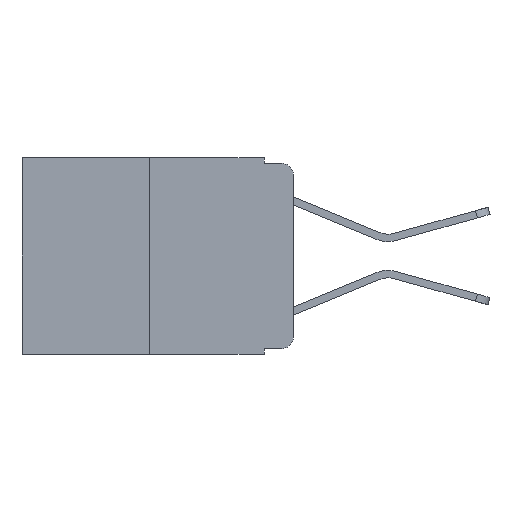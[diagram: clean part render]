
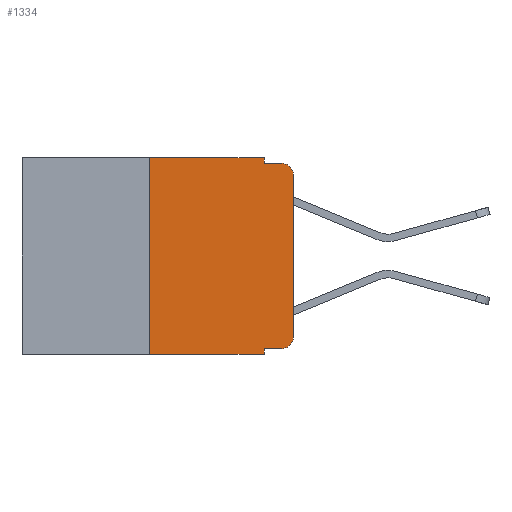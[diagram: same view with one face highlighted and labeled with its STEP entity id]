
A CAD part, left-side view. The second image highlights one B-rep face of the part: STEP entity #1334.
In plain terms, the highlighted planar face has unit normal (-1, 0, 0).
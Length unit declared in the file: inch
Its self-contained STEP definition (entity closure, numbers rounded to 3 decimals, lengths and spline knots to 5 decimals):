
#19 = VERTEX_POINT ( 'NONE', #2599 ) ;
#190 = EDGE_CURVE ( 'NONE', #11902, #3513, #4245, .T. ) ;
#820 = DIRECTION ( 'NONE',  ( 0., 0., 1. ) ) ;
#927 = LINE ( 'NONE', #3336, #10646 ) ;
#1154 = AXIS2_PLACEMENT_3D ( 'NONE', #10845, #9882, #5046 ) ;
#1334 = ADVANCED_FACE ( 'NONE', ( #6872 ), #12000, .F. ) ;
#1386 = ORIENTED_EDGE ( 'NONE', *, *, #3109, .F. ) ;
#1428 = CARTESIAN_POINT ( 'NONE',  ( 0., 0.02, -0.01 ) ) ;
#1674 = VECTOR ( 'NONE', #9749, 39.37008 ) ;
#1678 = CARTESIAN_POINT ( 'NONE',  ( 0., 0.051, -0.343 ) ) ;
#1734 = LINE ( 'NONE', #8211, #8474 ) ;
#1863 = CARTESIAN_POINT ( 'NONE',  ( 0., 0., 0. ) ) ;
#2050 = ORIENTED_EDGE ( 'NONE', *, *, #190, .T. ) ;
#2599 = CARTESIAN_POINT ( 'NONE',  ( 0., 0.051, -0.01 ) ) ;
#2748 = ORIENTED_EDGE ( 'NONE', *, *, #3443, .T. ) ;
#2886 = ORIENTED_EDGE ( 'NONE', *, *, #6286, .T. ) ;
#3109 = EDGE_CURVE ( 'NONE', #4150, #19, #5325, .T. ) ;
#3278 = ORIENTED_EDGE ( 'NONE', *, *, #6637, .T. ) ;
#3336 = CARTESIAN_POINT ( 'NONE',  ( 0., 0.051, -0.01 ) ) ;
#3443 = EDGE_CURVE ( 'NONE', #11919, #6403, #3807, .T. ) ;
#3448 = DIRECTION ( 'NONE',  ( 0., 0., -1. ) ) ;
#3478 = ORIENTED_EDGE ( 'NONE', *, *, #5490, .T. ) ;
#3513 = VERTEX_POINT ( 'NONE', #3883 ) ;
#3549 = VECTOR ( 'NONE', #4869, 39.37008 ) ;
#3807 = LINE ( 'NONE', #1863, #8863 ) ;
#3883 = CARTESIAN_POINT ( 'NONE',  ( 0., 0.02, -0.333 ) ) ;
#4150 = VERTEX_POINT ( 'NONE', #8395 ) ;
#4245 = LINE ( 'NONE', #9268, #1674 ) ;
#4333 = CARTESIAN_POINT ( 'NONE',  ( 0., 0.25, 0. ) ) ;
#4869 = DIRECTION ( 'NONE',  ( 0., -1., 0. ) ) ;
#5046 = DIRECTION ( 'NONE',  ( 0., 0., -1. ) ) ;
#5213 = CARTESIAN_POINT ( 'NONE',  ( 0., 0.02, -0.313 ) ) ;
#5229 = ORIENTED_EDGE ( 'NONE', *, *, #9604, .F. ) ;
#5242 = CIRCLE ( 'NONE', #10303, 0.02 ) ;
#5325 = LINE ( 'NONE', #10603, #7561 ) ;
#5409 = CARTESIAN_POINT ( 'NONE',  ( 0., 0.02, -0.03 ) ) ;
#5490 = EDGE_CURVE ( 'NONE', #6403, #6719, #7069, .T. ) ;
#5655 = DIRECTION ( 'NONE',  ( 0., -1., 0. ) ) ;
#5732 = LINE ( 'NONE', #7507, #7343 ) ;
#5844 = CARTESIAN_POINT ( 'NONE',  ( 0., 0., -0.313 ) ) ;
#5920 = LINE ( 'NONE', #4333, #8094 ) ;
#6179 = DIRECTION ( 'NONE',  ( 0., 0., -1. ) ) ;
#6286 = EDGE_CURVE ( 'NONE', #9713, #6885, #5732, .T. ) ;
#6373 = DIRECTION ( 'NONE',  ( 0., 0., -1. ) ) ;
#6403 = VERTEX_POINT ( 'NONE', #9488 ) ;
#6474 = ORIENTED_EDGE ( 'NONE', *, *, #9823, .F. ) ;
#6637 = EDGE_CURVE ( 'NONE', #3513, #11919, #5242, .T. ) ;
#6719 = VERTEX_POINT ( 'NONE', #1428 ) ;
#6762 = EDGE_CURVE ( 'NONE', #11902, #6885, #1734, .T. ) ;
#6872 = FACE_OUTER_BOUND ( 'NONE', #8983, .T. ) ;
#6885 = VERTEX_POINT ( 'NONE', #1678 ) ;
#7069 = CIRCLE ( 'NONE', #9379, 0.02 ) ;
#7343 = VECTOR ( 'NONE', #5655, 39.37008 ) ;
#7471 = VERTEX_POINT ( 'NONE', #9472 ) ;
#7507 = CARTESIAN_POINT ( 'NONE',  ( 0., 0.473, -0.343 ) ) ;
#7561 = VECTOR ( 'NONE', #10616, 39.37008 ) ;
#8094 = VECTOR ( 'NONE', #10849, 39.37008 ) ;
#8211 = CARTESIAN_POINT ( 'NONE',  ( 0., 0.051, 0. ) ) ;
#8395 = CARTESIAN_POINT ( 'NONE',  ( 0., 0.051, 0. ) ) ;
#8474 = VECTOR ( 'NONE', #3448, 39.37008 ) ;
#8863 = VECTOR ( 'NONE', #820, 39.37008 ) ;
#8983 = EDGE_LOOP ( 'NONE', ( #2748, #3478, #5229, #1386, #9545, #6474, #2886, #9795, #2050, #3278 ) ) ;
#9268 = CARTESIAN_POINT ( 'NONE',  ( 0., 0.051, -0.333 ) ) ;
#9379 = AXIS2_PLACEMENT_3D ( 'NONE', #5409, #11829, #6373 ) ;
#9472 = CARTESIAN_POINT ( 'NONE',  ( 0., 0.25, 0. ) ) ;
#9488 = CARTESIAN_POINT ( 'NONE',  ( 0., 0., -0.03 ) ) ;
#9545 = ORIENTED_EDGE ( 'NONE', *, *, #11918, .F. ) ;
#9604 = EDGE_CURVE ( 'NONE', #19, #6719, #927, .T. ) ;
#9713 = VERTEX_POINT ( 'NONE', #10956 ) ;
#9749 = DIRECTION ( 'NONE',  ( 0., -1., 0. ) ) ;
#9795 = ORIENTED_EDGE ( 'NONE', *, *, #6762, .F. ) ;
#9823 = EDGE_CURVE ( 'NONE', #9713, #7471, #5920, .T. ) ;
#9882 = DIRECTION ( 'NONE',  ( 1., 0., 0. ) ) ;
#9930 = DIRECTION ( 'NONE',  ( 0., -1., 0. ) ) ;
#10303 = AXIS2_PLACEMENT_3D ( 'NONE', #5213, #11648, #6179 ) ;
#10455 = LINE ( 'NONE', #11320, #3549 ) ;
#10603 = CARTESIAN_POINT ( 'NONE',  ( 0., 0.051, 0. ) ) ;
#10616 = DIRECTION ( 'NONE',  ( 0., 0., -1. ) ) ;
#10646 = VECTOR ( 'NONE', #9930, 39.37008 ) ;
#10845 = CARTESIAN_POINT ( 'NONE',  ( 0., 0.473, 0. ) ) ;
#10849 = DIRECTION ( 'NONE',  ( 0., 0., 1. ) ) ;
#10956 = CARTESIAN_POINT ( 'NONE',  ( 0., 0.25, -0.343 ) ) ;
#11320 = CARTESIAN_POINT ( 'NONE',  ( 0., 0.473, 0. ) ) ;
#11648 = DIRECTION ( 'NONE',  ( -1., 0., 0. ) ) ;
#11829 = DIRECTION ( 'NONE',  ( -1., 0., 0. ) ) ;
#11902 = VERTEX_POINT ( 'NONE', #12168 ) ;
#11918 = EDGE_CURVE ( 'NONE', #7471, #4150, #10455, .T. ) ;
#11919 = VERTEX_POINT ( 'NONE', #5844 ) ;
#12000 = PLANE ( 'NONE',  #1154 ) ;
#12168 = CARTESIAN_POINT ( 'NONE',  ( 0., 0.051, -0.333 ) ) ;
